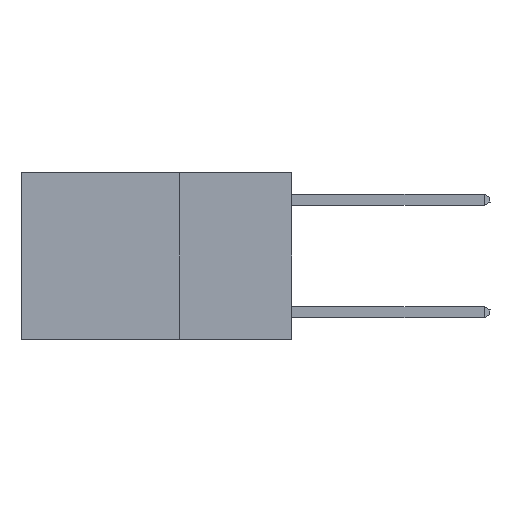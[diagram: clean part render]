
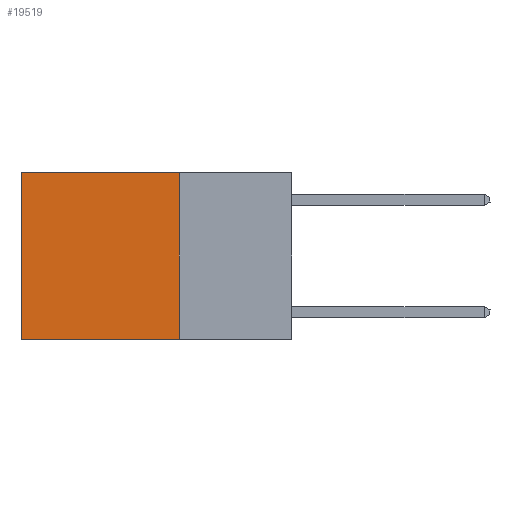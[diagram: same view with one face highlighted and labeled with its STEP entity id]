
A CAD part, left-side view. The second image highlights one B-rep face of the part: STEP entity #19519.
In plain terms, the highlighted planar face has unit normal (-1, 0, 0).
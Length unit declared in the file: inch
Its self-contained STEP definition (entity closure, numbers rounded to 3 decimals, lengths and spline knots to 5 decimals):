
#231 = VERTEX_POINT ( 'NONE', #13330 ) ;
#4689 = EDGE_CURVE ( 'NONE', #5090, #14933, #15956, .T. ) ;
#5090 = VERTEX_POINT ( 'NONE', #23653 ) ;
#5834 = CARTESIAN_POINT ( 'NONE',  ( 0.2625, 0.25, 0. ) ) ;
#6632 = CARTESIAN_POINT ( 'NONE',  ( 0.2625, 0.25, -0.37 ) ) ;
#6872 = VECTOR ( 'NONE', #14095, 39.37008 ) ;
#7395 = ORIENTED_EDGE ( 'NONE', *, *, #4689, .F. ) ;
#8231 = PLANE ( 'NONE',  #15070 ) ;
#10414 = CARTESIAN_POINT ( 'NONE',  ( 0.2625, 0.6, 0. ) ) ;
#10809 = CARTESIAN_POINT ( 'NONE',  ( 0.2625, 0.25, 0. ) ) ;
#11224 = DIRECTION ( 'NONE',  ( 0., 1., 0. ) ) ;
#13027 = LINE ( 'NONE', #5834, #18595 ) ;
#13330 = CARTESIAN_POINT ( 'NONE',  ( 0.2625, 0.25, 0. ) ) ;
#14095 = DIRECTION ( 'NONE',  ( 0., 1., 0. ) ) ;
#14385 = EDGE_LOOP ( 'NONE', ( #21553, #7395, #23783, #25109 ) ) ;
#14503 = VERTEX_POINT ( 'NONE', #10414 ) ;
#14742 = DIRECTION ( 'NONE',  ( 0., 0., -1. ) ) ;
#14933 = VERTEX_POINT ( 'NONE', #23680 ) ;
#15070 = AXIS2_PLACEMENT_3D ( 'NONE', #10809, #15387, #24715 ) ;
#15387 = DIRECTION ( 'NONE',  ( 1., 0., 0. ) ) ;
#15956 = LINE ( 'NONE', #6632, #28157 ) ;
#17282 = EDGE_CURVE ( 'NONE', #231, #5090, #13027, .T. ) ;
#17992 = EDGE_CURVE ( 'NONE', #14503, #14933, #26821, .T. ) ;
#18257 = EDGE_CURVE ( 'NONE', #231, #14503, #20662, .T. ) ;
#18595 = VECTOR ( 'NONE', #26781, 39.37008 ) ;
#19519 = ADVANCED_FACE ( 'NONE', ( #22112 ), #8231, .F. ) ;
#20662 = LINE ( 'NONE', #30018, #6872 ) ;
#21553 = ORIENTED_EDGE ( 'NONE', *, *, #17992, .T. ) ;
#22112 = FACE_OUTER_BOUND ( 'NONE', #14385, .T. ) ;
#23653 = CARTESIAN_POINT ( 'NONE',  ( 0.2625, 0.25, -0.37 ) ) ;
#23680 = CARTESIAN_POINT ( 'NONE',  ( 0.2625, 0.6, -0.37 ) ) ;
#23783 = ORIENTED_EDGE ( 'NONE', *, *, #17282, .F. ) ;
#24715 = DIRECTION ( 'NONE',  ( 0., 0., -1. ) ) ;
#25109 = ORIENTED_EDGE ( 'NONE', *, *, #18257, .T. ) ;
#26214 = CARTESIAN_POINT ( 'NONE',  ( 0.2625, 0.6, 0. ) ) ;
#26781 = DIRECTION ( 'NONE',  ( 0., 0., -1. ) ) ;
#26821 = LINE ( 'NONE', #26214, #29324 ) ;
#28157 = VECTOR ( 'NONE', #11224, 39.37008 ) ;
#29324 = VECTOR ( 'NONE', #14742, 39.37008 ) ;
#30018 = CARTESIAN_POINT ( 'NONE',  ( 0.2625, 0.25, 0. ) ) ;
